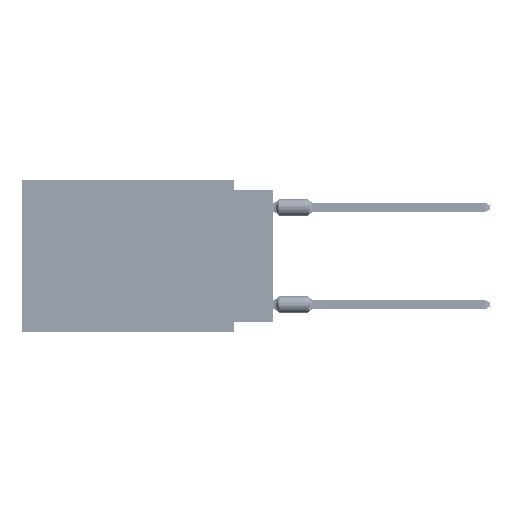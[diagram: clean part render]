
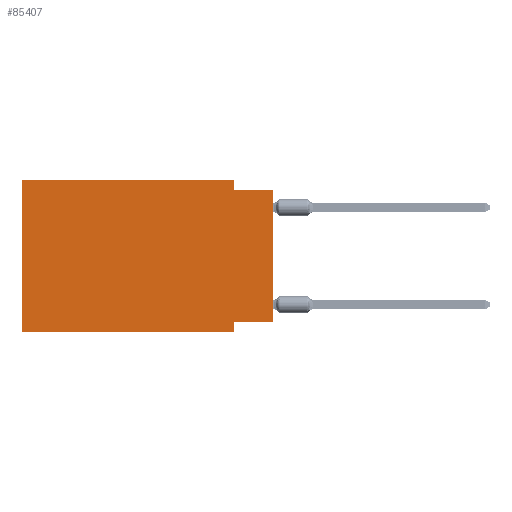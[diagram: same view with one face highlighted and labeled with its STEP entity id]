
A CAD part, left-side view. The second image highlights one B-rep face of the part: STEP entity #85407.
In plain terms, the highlighted planar face has unit normal (-1, 0, 0).
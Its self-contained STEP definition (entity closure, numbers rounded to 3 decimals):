
#975 = PLANE ( 'NONE',  #18018 ) ;
#2254 = ORIENTED_EDGE ( 'NONE', *, *, #73218, .F. ) ;
#2269 = DIRECTION ( 'NONE',  ( 0., 0., -1. ) ) ;
#2401 = VECTOR ( 'NONE', #19741, 1000. ) ;
#3246 = ORIENTED_EDGE ( 'NONE', *, *, #79472, .F. ) ;
#3536 = EDGE_CURVE ( 'NONE', #59270, #54902, #80194, .T. ) ;
#5597 = VECTOR ( 'NONE', #68230, 1000. ) ;
#8329 = EDGE_LOOP ( 'NONE', ( #85665, #60237, #3246, #21103, #42342, #20508, #17917, #2254 ) ) ;
#8884 = DIRECTION ( 'NONE',  ( 0., -1., 0. ) ) ;
#11180 = LINE ( 'NONE', #38982, #26593 ) ;
#12523 = EDGE_CURVE ( 'NONE', #28200, #79424, #73249, .T. ) ;
#14496 = LINE ( 'NONE', #41425, #47364 ) ;
#14747 = CARTESIAN_POINT ( 'NONE',  ( 0., 2.54, 0. ) ) ;
#15169 = DIRECTION ( 'NONE',  ( 0., 0., 1. ) ) ;
#15322 = EDGE_CURVE ( 'NONE', #79424, #46467, #14496, .T. ) ;
#15535 = DIRECTION ( 'NONE',  ( 1., 0., 0. ) ) ;
#17917 = ORIENTED_EDGE ( 'NONE', *, *, #3536, .F. ) ;
#18018 = AXIS2_PLACEMENT_3D ( 'NONE', #21713, #15535, #2269 ) ;
#19432 = CARTESIAN_POINT ( 'NONE',  ( 0., 2.54, -0.635 ) ) ;
#19741 = DIRECTION ( 'NONE',  ( 0., 0., -1. ) ) ;
#20417 = VERTEX_POINT ( 'NONE', #49804 ) ;
#20508 = ORIENTED_EDGE ( 'NONE', *, *, #24788, .T. ) ;
#20580 = CARTESIAN_POINT ( 'NONE',  ( 0., 16.383, 0. ) ) ;
#21018 = CARTESIAN_POINT ( 'NONE',  ( 0., 2.54, 0. ) ) ;
#21103 = ORIENTED_EDGE ( 'NONE', *, *, #15322, .F. ) ;
#21371 = CARTESIAN_POINT ( 'NONE',  ( 0., 0., 0. ) ) ;
#21713 = CARTESIAN_POINT ( 'NONE',  ( 0., 16.383, 0. ) ) ;
#24710 = CARTESIAN_POINT ( 'NONE',  ( 0., 16.383, -9.906 ) ) ;
#24731 = DIRECTION ( 'NONE',  ( 0., 0., 1. ) ) ;
#24788 = EDGE_CURVE ( 'NONE', #28200, #54902, #11180, .T. ) ;
#26593 = VECTOR ( 'NONE', #79138, 1000. ) ;
#26643 = CARTESIAN_POINT ( 'NONE',  ( 0., 0., -0.635 ) ) ;
#26719 = CARTESIAN_POINT ( 'NONE',  ( 0., 0., -0.635 ) ) ;
#28200 = VERTEX_POINT ( 'NONE', #24710 ) ;
#34322 = VECTOR ( 'NONE', #24731, 1000. ) ;
#35574 = LINE ( 'NONE', #81500, #82537 ) ;
#38982 = CARTESIAN_POINT ( 'NONE',  ( 0., 16.383, -9.906 ) ) ;
#41365 = EDGE_CURVE ( 'NONE', #75615, #77969, #67320, .T. ) ;
#41425 = CARTESIAN_POINT ( 'NONE',  ( 0., 16.383, 0. ) ) ;
#41580 = FACE_OUTER_BOUND ( 'NONE', #8329, .T. ) ;
#42100 = CARTESIAN_POINT ( 'NONE',  ( 0., 2.54, -9.906 ) ) ;
#42342 = ORIENTED_EDGE ( 'NONE', *, *, #12523, .F. ) ;
#44856 = VECTOR ( 'NONE', #15169, 1000. ) ;
#45896 = CARTESIAN_POINT ( 'NONE',  ( 0., 16.383, 0. ) ) ;
#46467 = VERTEX_POINT ( 'NONE', #14747 ) ;
#47364 = VECTOR ( 'NONE', #68353, 1000. ) ;
#49594 = LINE ( 'NONE', #21371, #44856 ) ;
#49804 = CARTESIAN_POINT ( 'NONE',  ( 0., 0., -9.271 ) ) ;
#54550 = LINE ( 'NONE', #21018, #5597 ) ;
#54902 = VERTEX_POINT ( 'NONE', #64664 ) ;
#56338 = EDGE_CURVE ( 'NONE', #20417, #77969, #49594, .T. ) ;
#59270 = VERTEX_POINT ( 'NONE', #81144 ) ;
#60237 = ORIENTED_EDGE ( 'NONE', *, *, #41365, .F. ) ;
#64664 = CARTESIAN_POINT ( 'NONE',  ( 0., 2.54, -9.906 ) ) ;
#67320 = LINE ( 'NONE', #26719, #80674 ) ;
#68230 = DIRECTION ( 'NONE',  ( 0., 0., -1. ) ) ;
#68259 = DIRECTION ( 'NONE',  ( 0., 1., 0. ) ) ;
#68353 = DIRECTION ( 'NONE',  ( 0., -1., 0. ) ) ;
#73218 = EDGE_CURVE ( 'NONE', #20417, #59270, #35574, .T. ) ;
#73249 = LINE ( 'NONE', #45896, #34322 ) ;
#75615 = VERTEX_POINT ( 'NONE', #19432 ) ;
#77969 = VERTEX_POINT ( 'NONE', #26643 ) ;
#79138 = DIRECTION ( 'NONE',  ( 0., -1., 0. ) ) ;
#79424 = VERTEX_POINT ( 'NONE', #20580 ) ;
#79472 = EDGE_CURVE ( 'NONE', #46467, #75615, #54550, .T. ) ;
#80194 = LINE ( 'NONE', #42100, #2401 ) ;
#80674 = VECTOR ( 'NONE', #8884, 1000. ) ;
#81144 = CARTESIAN_POINT ( 'NONE',  ( 0., 2.54, -9.271 ) ) ;
#81500 = CARTESIAN_POINT ( 'NONE',  ( 0., 0., -9.271 ) ) ;
#82537 = VECTOR ( 'NONE', #68259, 1000. ) ;
#85407 = ADVANCED_FACE ( 'NONE', ( #41580 ), #975, .F. ) ;
#85665 = ORIENTED_EDGE ( 'NONE', *, *, #56338, .T. ) ;
